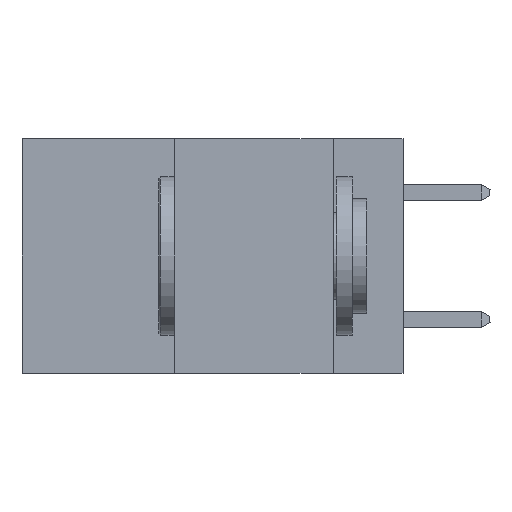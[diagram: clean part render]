
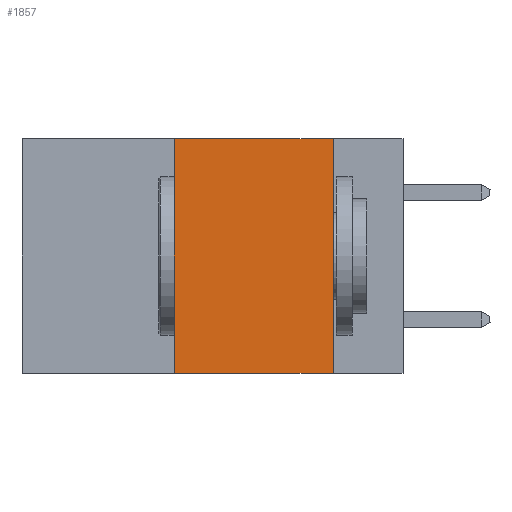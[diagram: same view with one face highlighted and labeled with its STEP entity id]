
A CAD part, left-side view. The second image highlights one B-rep face of the part: STEP entity #1857.
In plain terms, the highlighted planar face has unit normal (-1, 0, 0).
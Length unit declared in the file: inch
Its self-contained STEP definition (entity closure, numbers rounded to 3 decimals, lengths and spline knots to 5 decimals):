
#211 = EDGE_CURVE ( 'NONE', #1989, #9568, #573, .T. ) ;
#271 = ORIENTED_EDGE ( 'NONE', *, *, #211, .F. ) ;
#573 = LINE ( 'NONE', #7910, #2957 ) ;
#1211 = PLANE ( 'NONE',  #4259 ) ;
#1304 = EDGE_CURVE ( 'NONE', #1395, #8358, #7029, .T. ) ;
#1379 = CARTESIAN_POINT ( 'NONE',  ( 0., 0.11, 0. ) ) ;
#1395 = VERTEX_POINT ( 'NONE', #1379 ) ;
#1857 = ADVANCED_FACE ( 'NONE', ( #9168 ), #1211, .F. ) ;
#1989 = VERTEX_POINT ( 'NONE', #6628 ) ;
#2174 = ORIENTED_EDGE ( 'NONE', *, *, #1304, .F. ) ;
#2216 = VECTOR ( 'NONE', #7825, 39.37008 ) ;
#2229 = CARTESIAN_POINT ( 'NONE',  ( 0., 0.6, -0.37 ) ) ;
#2846 = LINE ( 'NONE', #2229, #2216 ) ;
#2957 = VECTOR ( 'NONE', #6310, 39.37008 ) ;
#3651 = VECTOR ( 'NONE', #8539, 39.37008 ) ;
#4259 = AXIS2_PLACEMENT_3D ( 'NONE', #5360, #8474, #4565 ) ;
#4425 = EDGE_CURVE ( 'NONE', #1989, #8358, #2846, .T. ) ;
#4565 = DIRECTION ( 'NONE',  ( 0., 0., -1. ) ) ;
#4624 = CARTESIAN_POINT ( 'NONE',  ( 0., 0.11, -0.37 ) ) ;
#5090 = LINE ( 'NONE', #8726, #7210 ) ;
#5360 = CARTESIAN_POINT ( 'NONE',  ( 0., 0.6, 0. ) ) ;
#5583 = EDGE_LOOP ( 'NONE', ( #2174, #7564, #271, #7927 ) ) ;
#6310 = DIRECTION ( 'NONE',  ( 0., 0., 1. ) ) ;
#6628 = CARTESIAN_POINT ( 'NONE',  ( 0., 0.36, -0.37 ) ) ;
#7029 = LINE ( 'NONE', #10153, #3651 ) ;
#7210 = VECTOR ( 'NONE', #10300, 39.37008 ) ;
#7564 = ORIENTED_EDGE ( 'NONE', *, *, #8099, .F. ) ;
#7825 = DIRECTION ( 'NONE',  ( 0., -1., 0. ) ) ;
#7910 = CARTESIAN_POINT ( 'NONE',  ( 0., 0.36, 0. ) ) ;
#7927 = ORIENTED_EDGE ( 'NONE', *, *, #4425, .T. ) ;
#8099 = EDGE_CURVE ( 'NONE', #9568, #1395, #5090, .T. ) ;
#8358 = VERTEX_POINT ( 'NONE', #4624 ) ;
#8474 = DIRECTION ( 'NONE',  ( 1., 0., 0. ) ) ;
#8539 = DIRECTION ( 'NONE',  ( 0., 0., -1. ) ) ;
#8726 = CARTESIAN_POINT ( 'NONE',  ( 0., 0.6, 0. ) ) ;
#9168 = FACE_OUTER_BOUND ( 'NONE', #5583, .T. ) ;
#9568 = VERTEX_POINT ( 'NONE', #9578 ) ;
#9578 = CARTESIAN_POINT ( 'NONE',  ( 0., 0.36, 0. ) ) ;
#10153 = CARTESIAN_POINT ( 'NONE',  ( 0., 0.11, 0. ) ) ;
#10300 = DIRECTION ( 'NONE',  ( 0., -1., 0. ) ) ;
